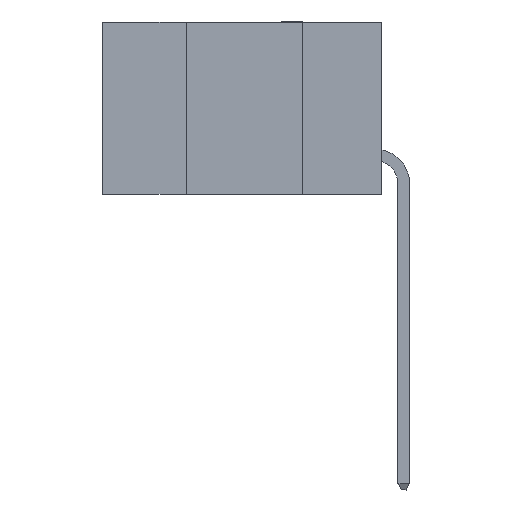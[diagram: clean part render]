
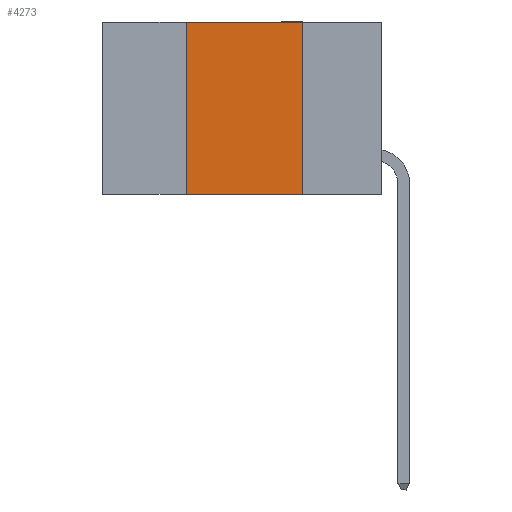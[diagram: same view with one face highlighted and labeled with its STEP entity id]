
A CAD part, left-side view. The second image highlights one B-rep face of the part: STEP entity #4273.
In plain terms, the highlighted planar face has unit normal (-1, 0, 0).
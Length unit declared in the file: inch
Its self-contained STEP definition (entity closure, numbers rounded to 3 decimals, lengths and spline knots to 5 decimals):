
#480 = CARTESIAN_POINT ( 'NONE',  ( 0., 0.17, 0. ) ) ;
#734 = VERTEX_POINT ( 'NONE', #3356 ) ;
#1875 = CARTESIAN_POINT ( 'NONE',  ( 0., 0.6, -0.37 ) ) ;
#1982 = CARTESIAN_POINT ( 'NONE',  ( 0., 0.6, 0. ) ) ;
#2647 = VECTOR ( 'NONE', #10007, 39.37008 ) ;
#2685 = DIRECTION ( 'NONE',  ( 0., -1., 0. ) ) ;
#2757 = VERTEX_POINT ( 'NONE', #6964 ) ;
#3101 = EDGE_LOOP ( 'NONE', ( #11770, #13550, #13431, #7597 ) ) ;
#3356 = CARTESIAN_POINT ( 'NONE',  ( 0., 0.42, -0.37 ) ) ;
#3864 = LINE ( 'NONE', #13646, #12741 ) ;
#3901 = DIRECTION ( 'NONE',  ( 0., -1., 0. ) ) ;
#4273 = ADVANCED_FACE ( 'NONE', ( #14034 ), #5613, .F. ) ;
#4630 = EDGE_CURVE ( 'NONE', #734, #11655, #9022, .T. ) ;
#5613 = PLANE ( 'NONE',  #8843 ) ;
#5833 = VECTOR ( 'NONE', #11468, 39.37008 ) ;
#6469 = LINE ( 'NONE', #480, #2647 ) ;
#6564 = DIRECTION ( 'NONE',  ( 1., 0., 0. ) ) ;
#6791 = EDGE_CURVE ( 'NONE', #2757, #9623, #3864, .T. ) ;
#6964 = CARTESIAN_POINT ( 'NONE',  ( 0., 0.42, 0. ) ) ;
#7597 = ORIENTED_EDGE ( 'NONE', *, *, #4630, .T. ) ;
#8033 = EDGE_CURVE ( 'NONE', #734, #2757, #13992, .T. ) ;
#8843 = AXIS2_PLACEMENT_3D ( 'NONE', #1982, #6564, #9137 ) ;
#9022 = LINE ( 'NONE', #1875, #14903 ) ;
#9137 = DIRECTION ( 'NONE',  ( 0., 0., -1. ) ) ;
#9623 = VERTEX_POINT ( 'NONE', #13416 ) ;
#10007 = DIRECTION ( 'NONE',  ( 0., 0., -1. ) ) ;
#11468 = DIRECTION ( 'NONE',  ( 0., 0., 1. ) ) ;
#11655 = VERTEX_POINT ( 'NONE', #11813 ) ;
#11770 = ORIENTED_EDGE ( 'NONE', *, *, #12840, .F. ) ;
#11813 = CARTESIAN_POINT ( 'NONE',  ( 0., 0.17, -0.37 ) ) ;
#12741 = VECTOR ( 'NONE', #2685, 39.37008 ) ;
#12840 = EDGE_CURVE ( 'NONE', #9623, #11655, #6469, .T. ) ;
#13416 = CARTESIAN_POINT ( 'NONE',  ( 0., 0.17, 0. ) ) ;
#13431 = ORIENTED_EDGE ( 'NONE', *, *, #8033, .F. ) ;
#13550 = ORIENTED_EDGE ( 'NONE', *, *, #6791, .F. ) ;
#13646 = CARTESIAN_POINT ( 'NONE',  ( 0., 0.6, 0. ) ) ;
#13752 = CARTESIAN_POINT ( 'NONE',  ( 0., 0.42, 0. ) ) ;
#13992 = LINE ( 'NONE', #13752, #5833 ) ;
#14034 = FACE_OUTER_BOUND ( 'NONE', #3101, .T. ) ;
#14903 = VECTOR ( 'NONE', #3901, 39.37008 ) ;
